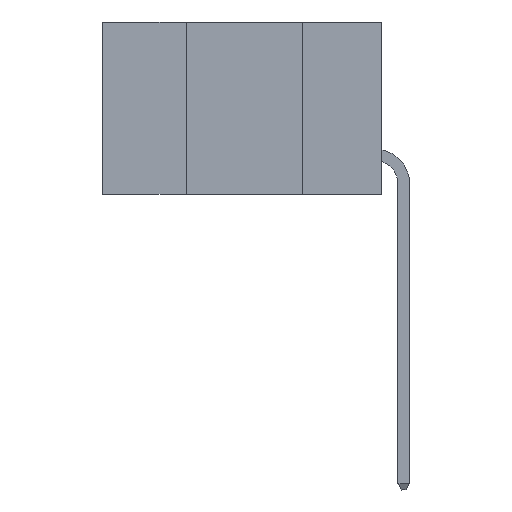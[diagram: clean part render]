
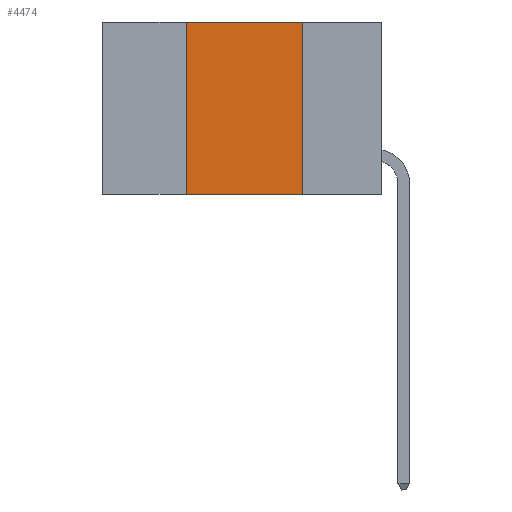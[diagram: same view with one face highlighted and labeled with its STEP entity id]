
A CAD part, left-side view. The second image highlights one B-rep face of the part: STEP entity #4474.
In plain terms, the highlighted planar face has unit normal (-1, 0, 0).
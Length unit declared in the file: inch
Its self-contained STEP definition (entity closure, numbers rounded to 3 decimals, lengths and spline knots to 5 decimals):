
#856 = CARTESIAN_POINT ( 'NONE',  ( 0., 0.6, 0. ) ) ;
#2274 = DIRECTION ( 'NONE',  ( 0., -1., 0. ) ) ;
#2535 = DIRECTION ( 'NONE',  ( 0., 0., -1. ) ) ;
#3377 = AXIS2_PLACEMENT_3D ( 'NONE', #13569, #10530, #14155 ) ;
#3685 = LINE ( 'NONE', #856, #10377 ) ;
#4474 = ADVANCED_FACE ( 'NONE', ( #7817 ), #14314, .F. ) ;
#6042 = VERTEX_POINT ( 'NONE', #15488 ) ;
#6044 = VECTOR ( 'NONE', #9338, 39.37008 ) ;
#6268 = LINE ( 'NONE', #9617, #11816 ) ;
#6545 = CARTESIAN_POINT ( 'NONE',  ( 0., 0.17, 0. ) ) ;
#6737 = LINE ( 'NONE', #6545, #15509 ) ;
#7189 = DIRECTION ( 'NONE',  ( 0., 0., 1. ) ) ;
#7616 = CARTESIAN_POINT ( 'NONE',  ( 0., 0.17, -0.37 ) ) ;
#7817 = FACE_OUTER_BOUND ( 'NONE', #9983, .T. ) ;
#8385 = EDGE_CURVE ( 'NONE', #10910, #12715, #3685, .T. ) ;
#9338 = DIRECTION ( 'NONE',  ( 0., -1., 0. ) ) ;
#9456 = EDGE_CURVE ( 'NONE', #12715, #12079, #6737, .T. ) ;
#9617 = CARTESIAN_POINT ( 'NONE',  ( 0., 0.42, 0. ) ) ;
#9723 = LINE ( 'NONE', #11595, #6044 ) ;
#9983 = EDGE_LOOP ( 'NONE', ( #10404, #11739, #11918, #11970 ) ) ;
#10335 = CARTESIAN_POINT ( 'NONE',  ( 0., 0.42, 0. ) ) ;
#10377 = VECTOR ( 'NONE', #2274, 39.37008 ) ;
#10404 = ORIENTED_EDGE ( 'NONE', *, *, #9456, .F. ) ;
#10530 = DIRECTION ( 'NONE',  ( 1., 0., 0. ) ) ;
#10889 = CARTESIAN_POINT ( 'NONE',  ( 0., 0.17, 0. ) ) ;
#10910 = VERTEX_POINT ( 'NONE', #10335 ) ;
#11595 = CARTESIAN_POINT ( 'NONE',  ( 0., 0.6, -0.37 ) ) ;
#11739 = ORIENTED_EDGE ( 'NONE', *, *, #8385, .F. ) ;
#11816 = VECTOR ( 'NONE', #7189, 39.37008 ) ;
#11828 = EDGE_CURVE ( 'NONE', #6042, #10910, #6268, .T. ) ;
#11918 = ORIENTED_EDGE ( 'NONE', *, *, #11828, .F. ) ;
#11970 = ORIENTED_EDGE ( 'NONE', *, *, #12408, .T. ) ;
#12079 = VERTEX_POINT ( 'NONE', #7616 ) ;
#12408 = EDGE_CURVE ( 'NONE', #6042, #12079, #9723, .T. ) ;
#12715 = VERTEX_POINT ( 'NONE', #10889 ) ;
#13569 = CARTESIAN_POINT ( 'NONE',  ( 0., 0.6, 0. ) ) ;
#14155 = DIRECTION ( 'NONE',  ( 0., 0., -1. ) ) ;
#14314 = PLANE ( 'NONE',  #3377 ) ;
#15488 = CARTESIAN_POINT ( 'NONE',  ( 0., 0.42, -0.37 ) ) ;
#15509 = VECTOR ( 'NONE', #2535, 39.37008 ) ;
